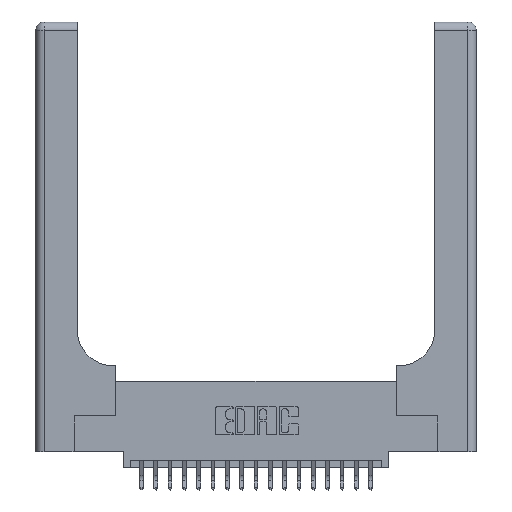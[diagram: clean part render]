
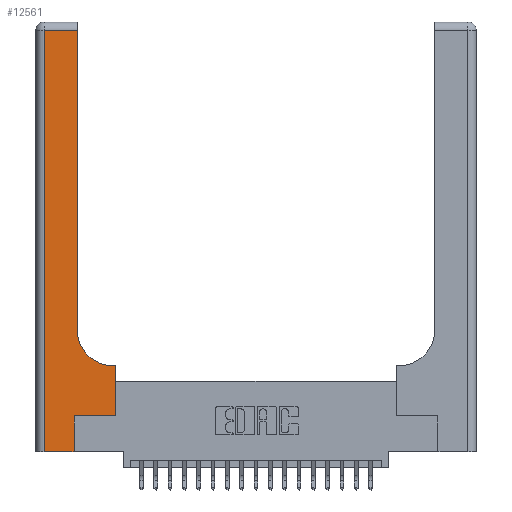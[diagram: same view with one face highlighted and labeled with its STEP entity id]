
A CAD part, top view. The second image highlights one B-rep face of the part: STEP entity #12561.
In plain terms, the highlighted planar face has unit normal (0, 0, 1).
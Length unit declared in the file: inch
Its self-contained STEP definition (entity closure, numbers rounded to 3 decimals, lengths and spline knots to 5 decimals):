
#708 = VERTEX_POINT ( 'NONE', #9559 ) ;
#929 = DIRECTION ( 'NONE',  ( 1., 0., 0. ) ) ;
#1196 = CIRCLE ( 'NONE', #18475, 0.25 ) ;
#1533 = CARTESIAN_POINT ( 'NONE',  ( 0.06, 3., 0.37 ) ) ;
#1674 = DIRECTION ( 'NONE',  ( 0., -1., 0. ) ) ;
#1734 = VECTOR ( 'NONE', #11266, 39.37008 ) ;
#1828 = VECTOR ( 'NONE', #4619, 39.37008 ) ;
#2130 = EDGE_CURVE ( 'NONE', #12054, #16283, #1196, .T. ) ;
#2360 = LINE ( 'NONE', #11386, #20329 ) ;
#2655 = LINE ( 'NONE', #11640, #1828 ) ;
#2911 = ORIENTED_EDGE ( 'NONE', *, *, #6223, .T. ) ;
#3474 = ORIENTED_EDGE ( 'NONE', *, *, #17141, .T. ) ;
#3581 = LINE ( 'NONE', #19295, #13470 ) ;
#3718 = VERTEX_POINT ( 'NONE', #9608 ) ;
#3836 = DIRECTION ( 'NONE',  ( 0., 1., 0. ) ) ;
#4048 = EDGE_CURVE ( 'NONE', #3718, #20137, #5899, .T. ) ;
#4177 = FACE_OUTER_BOUND ( 'NONE', #6668, .T. ) ;
#4619 = DIRECTION ( 'NONE',  ( -1., 0., 0. ) ) ;
#4681 = DIRECTION ( 'NONE',  ( 1., 0., 0. ) ) ;
#5071 = AXIS2_PLACEMENT_3D ( 'NONE', #6300, #20215, #6382 ) ;
#5175 = VECTOR ( 'NONE', #3836, 39.37008 ) ;
#5389 = CARTESIAN_POINT ( 'NONE',  ( 0.2915, 0.85, 0.37 ) ) ;
#5530 = DIRECTION ( 'NONE',  ( 0., 1., 0. ) ) ;
#5899 = LINE ( 'NONE', #1533, #20423 ) ;
#6223 = EDGE_CURVE ( 'NONE', #708, #7526, #9739, .T. ) ;
#6300 = CARTESIAN_POINT ( 'NONE',  ( 0., 3., 0.37 ) ) ;
#6371 = CARTESIAN_POINT ( 'NONE',  ( 0.5585, 0.6, 0.37 ) ) ;
#6382 = DIRECTION ( 'NONE',  ( -1., 0., 0. ) ) ;
#6668 = EDGE_LOOP ( 'NONE', ( #10510, #10934, #19132, #8877, #2911, #17663, #21103, #3474, #17767 ) ) ;
#7526 = VERTEX_POINT ( 'NONE', #16180 ) ;
#7680 = LINE ( 'NONE', #19676, #7956 ) ;
#7956 = VECTOR ( 'NONE', #929, 39.37008 ) ;
#8504 = LINE ( 'NONE', #13772, #16061 ) ;
#8877 = ORIENTED_EDGE ( 'NONE', *, *, #9378, .T. ) ;
#9034 = DIRECTION ( 'NONE',  ( 1., 0., 0. ) ) ;
#9378 = EDGE_CURVE ( 'NONE', #20137, #708, #8504, .T. ) ;
#9559 = CARTESIAN_POINT ( 'NONE',  ( 0.269, 0., 0.37 ) ) ;
#9608 = CARTESIAN_POINT ( 'NONE',  ( 0.06, 2.94, 0.37 ) ) ;
#9739 = LINE ( 'NONE', #20815, #5175 ) ;
#10167 = EDGE_CURVE ( 'NONE', #7526, #18323, #7680, .T. ) ;
#10285 = VERTEX_POINT ( 'NONE', #6371 ) ;
#10510 = ORIENTED_EDGE ( 'NONE', *, *, #10640, .T. ) ;
#10531 = CARTESIAN_POINT ( 'NONE',  ( 0.5415, 0.6, 0.37 ) ) ;
#10640 = EDGE_CURVE ( 'NONE', #16283, #18985, #2360, .T. ) ;
#10834 = LINE ( 'NONE', #13080, #1734 ) ;
#10934 = ORIENTED_EDGE ( 'NONE', *, *, #13400, .T. ) ;
#11266 = DIRECTION ( 'NONE',  ( -1., 0., 0. ) ) ;
#11386 = CARTESIAN_POINT ( 'NONE',  ( 0.2915, 3., 0.37 ) ) ;
#11640 = CARTESIAN_POINT ( 'NONE',  ( 0.2915, 0.6, 0.37 ) ) ;
#12054 = VERTEX_POINT ( 'NONE', #10531 ) ;
#12561 = ADVANCED_FACE ( 'NONE', ( #4177 ), #15251, .F. ) ;
#13080 = CARTESIAN_POINT ( 'NONE',  ( 0., 2.94, 0.37 ) ) ;
#13223 = CARTESIAN_POINT ( 'NONE',  ( 0.06, 0., 0.37 ) ) ;
#13400 = EDGE_CURVE ( 'NONE', #18985, #3718, #10834, .T. ) ;
#13470 = VECTOR ( 'NONE', #5530, 39.37008 ) ;
#13721 = CARTESIAN_POINT ( 'NONE',  ( 0.2915, 2.94, 0.37 ) ) ;
#13772 = CARTESIAN_POINT ( 'NONE',  ( 0., 0., 0.37 ) ) ;
#15251 = PLANE ( 'NONE',  #5071 ) ;
#15254 = DIRECTION ( 'NONE',  ( 0., 0., -1. ) ) ;
#16061 = VECTOR ( 'NONE', #9034, 39.37008 ) ;
#16180 = CARTESIAN_POINT ( 'NONE',  ( 0.269, 0.25, 0.37 ) ) ;
#16283 = VERTEX_POINT ( 'NONE', #5389 ) ;
#17141 = EDGE_CURVE ( 'NONE', #10285, #12054, #2655, .T. ) ;
#17663 = ORIENTED_EDGE ( 'NONE', *, *, #10167, .T. ) ;
#17767 = ORIENTED_EDGE ( 'NONE', *, *, #2130, .T. ) ;
#18148 = CARTESIAN_POINT ( 'NONE',  ( 0.5585, 0.25, 0.37 ) ) ;
#18323 = VERTEX_POINT ( 'NONE', #18148 ) ;
#18475 = AXIS2_PLACEMENT_3D ( 'NONE', #18630, #15254, #4681 ) ;
#18630 = CARTESIAN_POINT ( 'NONE',  ( 0.5415, 0.85, 0.37 ) ) ;
#18985 = VERTEX_POINT ( 'NONE', #13721 ) ;
#19132 = ORIENTED_EDGE ( 'NONE', *, *, #4048, .T. ) ;
#19295 = CARTESIAN_POINT ( 'NONE',  ( 0.5585, 0.25, 0.37 ) ) ;
#19676 = CARTESIAN_POINT ( 'NONE',  ( 0.269, 0.25, 0.37 ) ) ;
#19982 = DIRECTION ( 'NONE',  ( 0., 1., 0. ) ) ;
#20137 = VERTEX_POINT ( 'NONE', #13223 ) ;
#20215 = DIRECTION ( 'NONE',  ( 0., 0., -1. ) ) ;
#20329 = VECTOR ( 'NONE', #19982, 39.37008 ) ;
#20423 = VECTOR ( 'NONE', #1674, 39.37008 ) ;
#20815 = CARTESIAN_POINT ( 'NONE',  ( 0.269, 0., 0.37 ) ) ;
#21095 = EDGE_CURVE ( 'NONE', #18323, #10285, #3581, .T. ) ;
#21103 = ORIENTED_EDGE ( 'NONE', *, *, #21095, .T. ) ;
